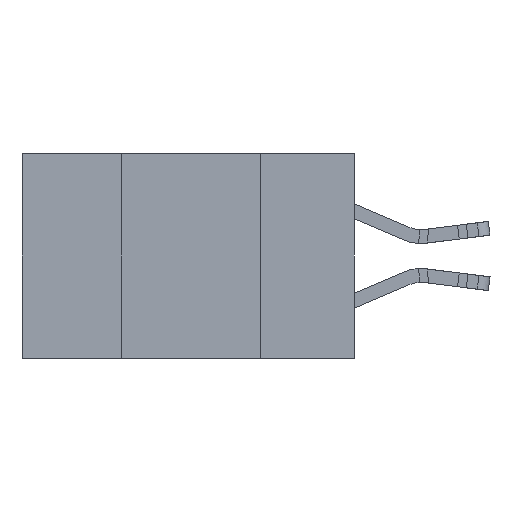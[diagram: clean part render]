
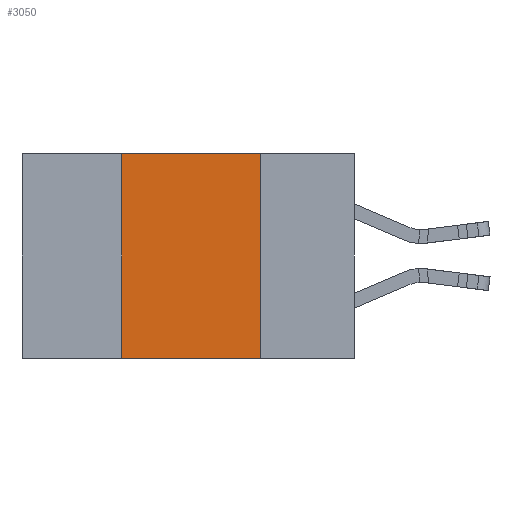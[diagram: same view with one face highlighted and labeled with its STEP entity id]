
A CAD part, left-side view. The second image highlights one B-rep face of the part: STEP entity #3050.
In plain terms, the highlighted planar face has unit normal (-1, 0, 0).
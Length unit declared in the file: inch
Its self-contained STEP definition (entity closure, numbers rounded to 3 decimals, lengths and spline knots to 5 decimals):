
#104 = VECTOR ( 'NONE', #11618, 39.37008 ) ;
#231 = ORIENTED_EDGE ( 'NONE', *, *, #5784, .F. ) ;
#363 = EDGE_CURVE ( 'NONE', #9830, #18753, #12839, .T. ) ;
#3050 = ADVANCED_FACE ( 'NONE', ( #5280 ), #21075, .F. ) ;
#3562 = VECTOR ( 'NONE', #14449, 39.37008 ) ;
#4009 = CARTESIAN_POINT ( 'NONE',  ( 0., 0.42, -0.37 ) ) ;
#5280 = FACE_OUTER_BOUND ( 'NONE', #17480, .T. ) ;
#5413 = VECTOR ( 'NONE', #8727, 39.37008 ) ;
#5784 = EDGE_CURVE ( 'NONE', #9830, #15812, #21471, .T. ) ;
#7137 = EDGE_CURVE ( 'NONE', #15812, #12514, #16116, .T. ) ;
#8486 = EDGE_CURVE ( 'NONE', #12514, #18753, #14232, .T. ) ;
#8511 = CARTESIAN_POINT ( 'NONE',  ( 0., 0.6, 0. ) ) ;
#8727 = DIRECTION ( 'NONE',  ( 0., -1., 0. ) ) ;
#9830 = VERTEX_POINT ( 'NONE', #4009 ) ;
#11322 = AXIS2_PLACEMENT_3D ( 'NONE', #21168, #20523, #20228 ) ;
#11588 = ORIENTED_EDGE ( 'NONE', *, *, #7137, .F. ) ;
#11618 = DIRECTION ( 'NONE',  ( 0., 0., 1. ) ) ;
#11649 = CARTESIAN_POINT ( 'NONE',  ( 0., 0.42, -0.37 ) ) ;
#12212 = ORIENTED_EDGE ( 'NONE', *, *, #8486, .F. ) ;
#12514 = VERTEX_POINT ( 'NONE', #16014 ) ;
#12839 = LINE ( 'NONE', #21488, #22843 ) ;
#14232 = LINE ( 'NONE', #14271, #3562 ) ;
#14271 = CARTESIAN_POINT ( 'NONE',  ( 0., 0.17, -0.37 ) ) ;
#14449 = DIRECTION ( 'NONE',  ( 0., 0., -1. ) ) ;
#15812 = VERTEX_POINT ( 'NONE', #17614 ) ;
#16014 = CARTESIAN_POINT ( 'NONE',  ( 0., 0.17, 0. ) ) ;
#16116 = LINE ( 'NONE', #8511, #5413 ) ;
#16124 = DIRECTION ( 'NONE',  ( 0., -1., 0. ) ) ;
#17480 = EDGE_LOOP ( 'NONE', ( #12212, #11588, #231, #20962 ) ) ;
#17614 = CARTESIAN_POINT ( 'NONE',  ( 0., 0.42, 0. ) ) ;
#17839 = CARTESIAN_POINT ( 'NONE',  ( 0., 0.17, -0.37 ) ) ;
#18753 = VERTEX_POINT ( 'NONE', #17839 ) ;
#20228 = DIRECTION ( 'NONE',  ( 0., 0., -1. ) ) ;
#20523 = DIRECTION ( 'NONE',  ( 1., 0., 0. ) ) ;
#20962 = ORIENTED_EDGE ( 'NONE', *, *, #363, .T. ) ;
#21075 = PLANE ( 'NONE',  #11322 ) ;
#21168 = CARTESIAN_POINT ( 'NONE',  ( 0., 0.6, 0. ) ) ;
#21471 = LINE ( 'NONE', #11649, #104 ) ;
#21488 = CARTESIAN_POINT ( 'NONE',  ( 0., 0.6, -0.37 ) ) ;
#22843 = VECTOR ( 'NONE', #16124, 39.37008 ) ;
